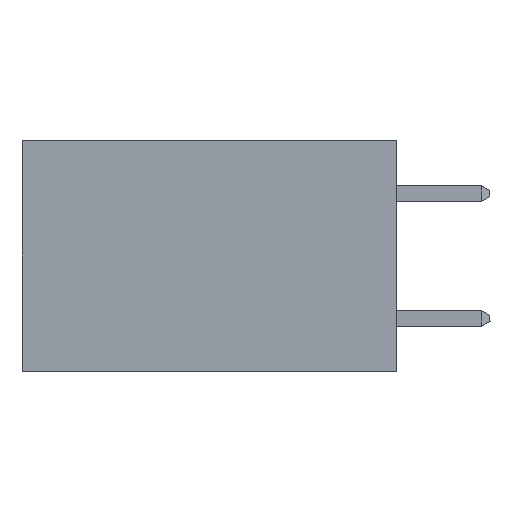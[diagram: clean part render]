
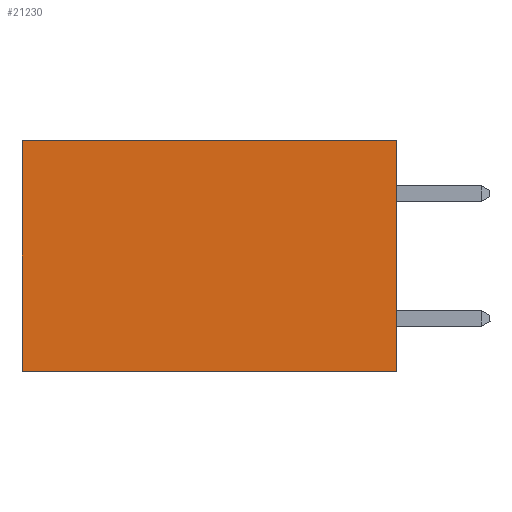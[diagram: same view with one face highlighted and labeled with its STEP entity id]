
A CAD part, left-side view. The second image highlights one B-rep face of the part: STEP entity #21230.
In plain terms, the highlighted planar face has unit normal (-1, 0, 0).
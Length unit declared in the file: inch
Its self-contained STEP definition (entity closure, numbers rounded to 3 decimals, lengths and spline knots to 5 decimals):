
#19 = VERTEX_POINT ( 'NONE', #12080 ) ;
#1090 = CARTESIAN_POINT ( 'NONE',  ( 0.298, 0., 0. ) ) ;
#1643 = CARTESIAN_POINT ( 'NONE',  ( 0.298, 0., 0. ) ) ;
#2794 = EDGE_CURVE ( 'NONE', #21253, #24901, #12529, .T. ) ;
#3382 = DIRECTION ( 'NONE',  ( 0., 0., -1. ) ) ;
#5267 = DIRECTION ( 'NONE',  ( 0., 1., 0. ) ) ;
#5546 = CARTESIAN_POINT ( 'NONE',  ( 0.298, 0., 0. ) ) ;
#6498 = FACE_OUTER_BOUND ( 'NONE', #24959, .T. ) ;
#8330 = LINE ( 'NONE', #1090, #25086 ) ;
#9534 = EDGE_CURVE ( 'NONE', #22366, #19, #8330, .T. ) ;
#9869 = DIRECTION ( 'NONE',  ( 1., 0., 0. ) ) ;
#11212 = VECTOR ( 'NONE', #16610, 39.37008 ) ;
#11339 = AXIS2_PLACEMENT_3D ( 'NONE', #5546, #9869, #20135 ) ;
#11799 = CARTESIAN_POINT ( 'NONE',  ( 0.298, 0., -0.37 ) ) ;
#11921 = CARTESIAN_POINT ( 'NONE',  ( 0.298, 0., 0. ) ) ;
#12080 = CARTESIAN_POINT ( 'NONE',  ( 0.298, 0., -0.37 ) ) ;
#12529 = LINE ( 'NONE', #20302, #11212 ) ;
#13165 = VECTOR ( 'NONE', #5267, 39.37008 ) ;
#13668 = ORIENTED_EDGE ( 'NONE', *, *, #9534, .F. ) ;
#14204 = CARTESIAN_POINT ( 'NONE',  ( 0.298, 0.6, 0. ) ) ;
#14801 = LINE ( 'NONE', #11799, #13165 ) ;
#15824 = LINE ( 'NONE', #1643, #23408 ) ;
#16106 = DIRECTION ( 'NONE',  ( 0., 1., 0. ) ) ;
#16337 = ORIENTED_EDGE ( 'NONE', *, *, #23103, .T. ) ;
#16610 = DIRECTION ( 'NONE',  ( 0., 0., -1. ) ) ;
#19313 = EDGE_CURVE ( 'NONE', #19, #24901, #14801, .T. ) ;
#20135 = DIRECTION ( 'NONE',  ( 0., 0., -1. ) ) ;
#20302 = CARTESIAN_POINT ( 'NONE',  ( 0.298, 0.6, 0. ) ) ;
#21230 = ADVANCED_FACE ( 'NONE', ( #6498 ), #26533, .F. ) ;
#21253 = VERTEX_POINT ( 'NONE', #14204 ) ;
#21746 = ORIENTED_EDGE ( 'NONE', *, *, #2794, .T. ) ;
#22366 = VERTEX_POINT ( 'NONE', #11921 ) ;
#22455 = ORIENTED_EDGE ( 'NONE', *, *, #19313, .F. ) ;
#23103 = EDGE_CURVE ( 'NONE', #22366, #21253, #15824, .T. ) ;
#23408 = VECTOR ( 'NONE', #16106, 39.37008 ) ;
#24901 = VERTEX_POINT ( 'NONE', #26047 ) ;
#24959 = EDGE_LOOP ( 'NONE', ( #21746, #22455, #13668, #16337 ) ) ;
#25086 = VECTOR ( 'NONE', #3382, 39.37008 ) ;
#26047 = CARTESIAN_POINT ( 'NONE',  ( 0.298, 0.6, -0.37 ) ) ;
#26533 = PLANE ( 'NONE',  #11339 ) ;
